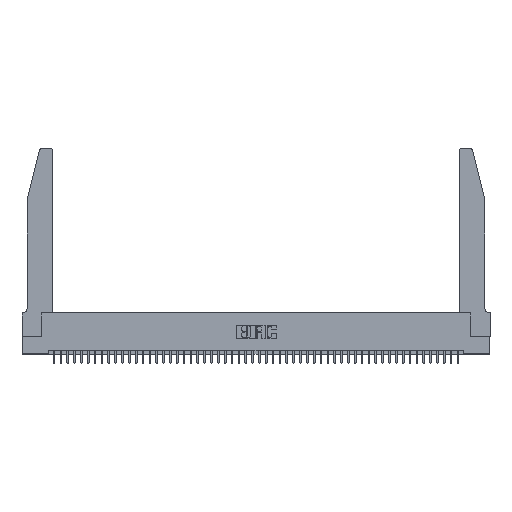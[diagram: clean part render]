
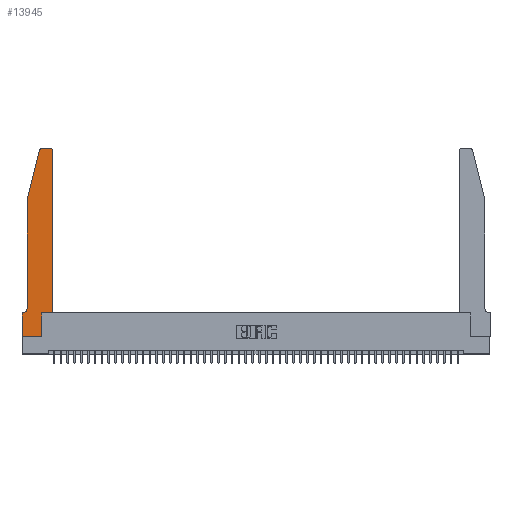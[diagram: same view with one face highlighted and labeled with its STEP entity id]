
A CAD part, top view. The second image highlights one B-rep face of the part: STEP entity #13945.
In plain terms, the highlighted planar face has unit normal (0, 0, 1).
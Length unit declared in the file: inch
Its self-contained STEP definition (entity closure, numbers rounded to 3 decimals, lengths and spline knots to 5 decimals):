
#136 = DIRECTION ( 'NONE',  ( 0., 0., -1. ) ) ;
#283 = EDGE_LOOP ( 'NONE', ( #5632, #36532, #36628, #20284, #39891, #25865, #44099, #33280, #13733, #28042, #48645, #13807 ) ) ;
#1223 = VERTEX_POINT ( 'NONE', #47883 ) ;
#1668 = DIRECTION ( 'NONE',  ( 1., 0., 0. ) ) ;
#2847 = CARTESIAN_POINT ( 'NONE',  ( 0.0755, 2., 0.37 ) ) ;
#5183 = CARTESIAN_POINT ( 'NONE',  ( 0.4505, 0.35, 0.37 ) ) ;
#5632 = ORIENTED_EDGE ( 'NONE', *, *, #32198, .T. ) ;
#5777 = VERTEX_POINT ( 'NONE', #24065 ) ;
#5858 = AXIS2_PLACEMENT_3D ( 'NONE', #15618, #22831, #19592 ) ;
#6498 = AXIS2_PLACEMENT_3D ( 'NONE', #20798, #43887, #1668 ) ;
#6628 = VECTOR ( 'NONE', #15786, 39.37008 ) ;
#6902 = CARTESIAN_POINT ( 'NONE',  ( 0.284, 2.75, 0.37 ) ) ;
#7020 = VECTOR ( 'NONE', #9247, 39.37008 ) ;
#7455 = EDGE_CURVE ( 'NONE', #26268, #31800, #32652, .T. ) ;
#7690 = EDGE_CURVE ( 'NONE', #31800, #11377, #14633, .T. ) ;
#8060 = EDGE_CURVE ( 'NONE', #31319, #28834, #29023, .T. ) ;
#8103 = CARTESIAN_POINT ( 'NONE',  ( 0.2865, 0., 0.37 ) ) ;
#8348 = EDGE_CURVE ( 'NONE', #45109, #38057, #19948, .T. ) ;
#9089 = CARTESIAN_POINT ( 'NONE',  ( 0.0755, 0.35, 0.37 ) ) ;
#9247 = DIRECTION ( 'NONE',  ( 1., 0., 0. ) ) ;
#10127 = CARTESIAN_POINT ( 'NONE',  ( 0., 0., 0.37 ) ) ;
#10214 = CARTESIAN_POINT ( 'NONE',  ( 0.2605, 2.75, 0.37 ) ) ;
#10365 = DIRECTION ( 'NONE',  ( -1., 0., 0. ) ) ;
#10877 = CARTESIAN_POINT ( 'NONE',  ( 0., 0., 0.37 ) ) ;
#11094 = VERTEX_POINT ( 'NONE', #30213 ) ;
#11309 = PLANE ( 'NONE',  #5858 ) ;
#11377 = VERTEX_POINT ( 'NONE', #10127 ) ;
#11577 = CARTESIAN_POINT ( 'NONE',  ( 0.4205, 2.72, 0.37 ) ) ;
#13241 = AXIS2_PLACEMENT_3D ( 'NONE', #42170, #136, #46693 ) ;
#13733 = ORIENTED_EDGE ( 'NONE', *, *, #34418, .T. ) ;
#13807 = ORIENTED_EDGE ( 'NONE', *, *, #20820, .T. ) ;
#13945 = ADVANCED_FACE ( 'NONE', ( #48226 ), #11309, .T. ) ;
#14037 = CARTESIAN_POINT ( 'NONE',  ( 0.2865, 0.35, 0.37 ) ) ;
#14633 = LINE ( 'NONE', #10877, #21851 ) ;
#15365 = DIRECTION ( 'NONE',  ( 0., 0., 1. ) ) ;
#15618 = CARTESIAN_POINT ( 'NONE',  ( 0., 0.35, 0.37 ) ) ;
#15675 = CARTESIAN_POINT ( 'NONE',  ( 0.4505, 2.72, 0.37 ) ) ;
#15786 = DIRECTION ( 'NONE',  ( 1., 0., 0. ) ) ;
#16105 = CARTESIAN_POINT ( 'NONE',  ( 0., 0., 0.37 ) ) ;
#17066 = VERTEX_POINT ( 'NONE', #6902 ) ;
#17217 = DIRECTION ( 'NONE',  ( -1., 0., 0. ) ) ;
#19592 = DIRECTION ( 'NONE',  ( 1., 0., 0. ) ) ;
#19821 = CIRCLE ( 'NONE', #23886, 0.03 ) ;
#19948 = LINE ( 'NONE', #40081, #46923 ) ;
#20215 = CARTESIAN_POINT ( 'NONE',  ( 0.4505, 0.35, 0.37 ) ) ;
#20284 = ORIENTED_EDGE ( 'NONE', *, *, #8348, .T. ) ;
#20798 = CARTESIAN_POINT ( 'NONE',  ( 0.284, 2.72, 0.37 ) ) ;
#20820 = EDGE_CURVE ( 'NONE', #28834, #11094, #19821, .T. ) ;
#20848 = LINE ( 'NONE', #2847, #46600 ) ;
#20968 = LINE ( 'NONE', #10214, #29350 ) ;
#21515 = DIRECTION ( 'NONE',  ( 0., -1., 0. ) ) ;
#21851 = VECTOR ( 'NONE', #41939, 39.37008 ) ;
#22831 = DIRECTION ( 'NONE',  ( 0., 0., 1. ) ) ;
#23256 = CARTESIAN_POINT ( 'NONE',  ( 0., 0.35, 0.37 ) ) ;
#23886 = AXIS2_PLACEMENT_3D ( 'NONE', #11577, #15365, #38301 ) ;
#23932 = VERTEX_POINT ( 'NONE', #8103 ) ;
#24065 = CARTESIAN_POINT ( 'NONE',  ( 0.25487, 2.72718, 0.37 ) ) ;
#25084 = EDGE_CURVE ( 'NONE', #11377, #23932, #45518, .T. ) ;
#25865 = ORIENTED_EDGE ( 'NONE', *, *, #7455, .T. ) ;
#26268 = VERTEX_POINT ( 'NONE', #34904 ) ;
#27184 = VECTOR ( 'NONE', #35249, 39.37008 ) ;
#27320 = EDGE_CURVE ( 'NONE', #17066, #5777, #35721, .T. ) ;
#27347 = LINE ( 'NONE', #20215, #7020 ) ;
#28042 = ORIENTED_EDGE ( 'NONE', *, *, #28173, .T. ) ;
#28173 = EDGE_CURVE ( 'NONE', #1223, #31319, #27347, .T. ) ;
#28834 = VERTEX_POINT ( 'NONE', #15675 ) ;
#29023 = LINE ( 'NONE', #5183, #27184 ) ;
#29350 = VECTOR ( 'NONE', #10365, 39.37008 ) ;
#30213 = CARTESIAN_POINT ( 'NONE',  ( 0.4205, 2.75, 0.37 ) ) ;
#31319 = VERTEX_POINT ( 'NONE', #38675 ) ;
#31524 = CARTESIAN_POINT ( 'NONE',  ( 0.0755, 2., 0.37 ) ) ;
#31800 = VERTEX_POINT ( 'NONE', #23256 ) ;
#32198 = EDGE_CURVE ( 'NONE', #11094, #17066, #20968, .T. ) ;
#32652 = LINE ( 'NONE', #9089, #42233 ) ;
#33280 = ORIENTED_EDGE ( 'NONE', *, *, #25084, .T. ) ;
#33425 = DIRECTION ( 'NONE',  ( 0., 1., 0. ) ) ;
#34113 = CIRCLE ( 'NONE', #13241, 0.07 ) ;
#34418 = EDGE_CURVE ( 'NONE', #23932, #1223, #48275, .T. ) ;
#34904 = CARTESIAN_POINT ( 'NONE',  ( 0.0055, 0.35, 0.37 ) ) ;
#35249 = DIRECTION ( 'NONE',  ( 0., 1., 0. ) ) ;
#35721 = CIRCLE ( 'NONE', #6498, 0.03 ) ;
#36532 = ORIENTED_EDGE ( 'NONE', *, *, #27320, .T. ) ;
#36628 = ORIENTED_EDGE ( 'NONE', *, *, #36938, .T. ) ;
#36938 = EDGE_CURVE ( 'NONE', #5777, #45109, #20848, .T. ) ;
#37200 = DIRECTION ( 'NONE',  ( -0.239, -0.971, 0. ) ) ;
#38041 = VECTOR ( 'NONE', #33425, 39.37008 ) ;
#38057 = VERTEX_POINT ( 'NONE', #43356 ) ;
#38301 = DIRECTION ( 'NONE',  ( 1., 0., 0. ) ) ;
#38675 = CARTESIAN_POINT ( 'NONE',  ( 0.4505, 0.35, 0.37 ) ) ;
#39891 = ORIENTED_EDGE ( 'NONE', *, *, #45601, .T. ) ;
#40081 = CARTESIAN_POINT ( 'NONE',  ( 0.0755, 2., 0.37 ) ) ;
#41939 = DIRECTION ( 'NONE',  ( 0., -1., 0. ) ) ;
#42170 = CARTESIAN_POINT ( 'NONE',  ( 0.0055, 0.42, 0.37 ) ) ;
#42233 = VECTOR ( 'NONE', #17217, 39.37008 ) ;
#43356 = CARTESIAN_POINT ( 'NONE',  ( 0.0755, 0.42, 0.37 ) ) ;
#43887 = DIRECTION ( 'NONE',  ( 0., 0., 1. ) ) ;
#44099 = ORIENTED_EDGE ( 'NONE', *, *, #7690, .T. ) ;
#45109 = VERTEX_POINT ( 'NONE', #31524 ) ;
#45518 = LINE ( 'NONE', #16105, #6628 ) ;
#45601 = EDGE_CURVE ( 'NONE', #38057, #26268, #34113, .T. ) ;
#46600 = VECTOR ( 'NONE', #37200, 39.37008 ) ;
#46693 = DIRECTION ( 'NONE',  ( -1., 0., 0. ) ) ;
#46923 = VECTOR ( 'NONE', #21515, 39.37008 ) ;
#47883 = CARTESIAN_POINT ( 'NONE',  ( 0.2865, 0.35, 0.37 ) ) ;
#48226 = FACE_OUTER_BOUND ( 'NONE', #283, .T. ) ;
#48275 = LINE ( 'NONE', #14037, #38041 ) ;
#48645 = ORIENTED_EDGE ( 'NONE', *, *, #8060, .T. ) ;
